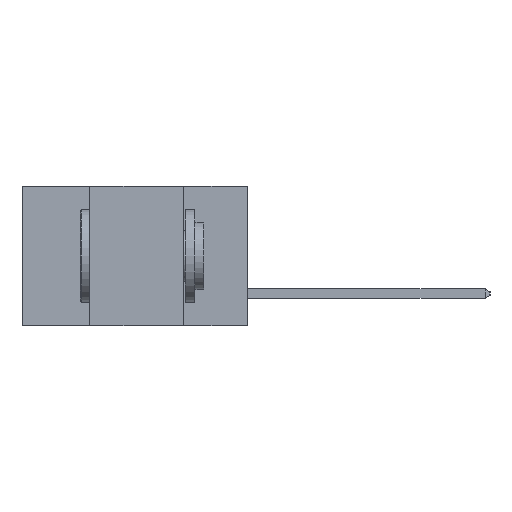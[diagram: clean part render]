
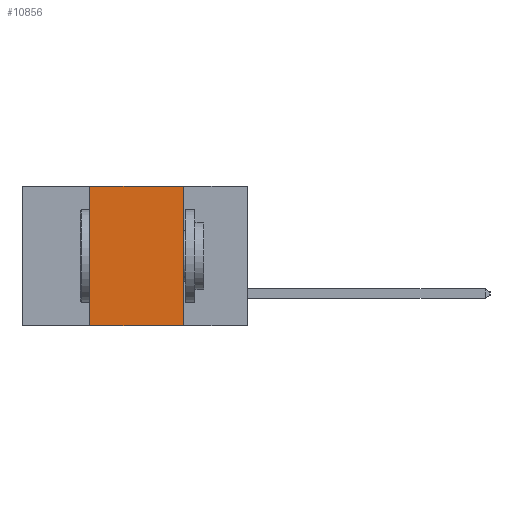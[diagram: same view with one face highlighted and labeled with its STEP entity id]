
A CAD part, left-side view. The second image highlights one B-rep face of the part: STEP entity #10856.
In plain terms, the highlighted planar face has unit normal (-1, 0, 0).
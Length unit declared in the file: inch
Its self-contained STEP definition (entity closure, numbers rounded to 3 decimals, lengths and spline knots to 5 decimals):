
#7 = CARTESIAN_POINT ( 'NONE',  ( 0., 0.6, 0. ) ) ;
#168 = ORIENTED_EDGE ( 'NONE', *, *, #8483, .F. ) ;
#930 = VECTOR ( 'NONE', #4495, 39.37008 ) ;
#2107 = CARTESIAN_POINT ( 'NONE',  ( 0., 0.17, 0. ) ) ;
#2740 = CARTESIAN_POINT ( 'NONE',  ( 0., 0.17, -0.37 ) ) ;
#2755 = DIRECTION ( 'NONE',  ( 0., 0., -1. ) ) ;
#2993 = EDGE_LOOP ( 'NONE', ( #13557, #168, #4222, #8613 ) ) ;
#3478 = EDGE_CURVE ( 'NONE', #11890, #4341, #4555, .T. ) ;
#3724 = VECTOR ( 'NONE', #5319, 39.37008 ) ;
#4222 = ORIENTED_EDGE ( 'NONE', *, *, #3478, .F. ) ;
#4341 = VERTEX_POINT ( 'NONE', #12393 ) ;
#4495 = DIRECTION ( 'NONE',  ( 0., 0., 1. ) ) ;
#4555 = LINE ( 'NONE', #6664, #930 ) ;
#5208 = CARTESIAN_POINT ( 'NONE',  ( 0., 0.42, -0.37 ) ) ;
#5319 = DIRECTION ( 'NONE',  ( 0., 0., -1. ) ) ;
#5603 = VERTEX_POINT ( 'NONE', #2740 ) ;
#6178 = EDGE_CURVE ( 'NONE', #11842, #5603, #11671, .T. ) ;
#6664 = CARTESIAN_POINT ( 'NONE',  ( 0., 0.42, 0. ) ) ;
#6954 = FACE_OUTER_BOUND ( 'NONE', #2993, .T. ) ;
#6997 = CARTESIAN_POINT ( 'NONE',  ( 0., 0.6, -0.37 ) ) ;
#7418 = VECTOR ( 'NONE', #13655, 39.37008 ) ;
#8483 = EDGE_CURVE ( 'NONE', #4341, #11842, #16281, .T. ) ;
#8613 = ORIENTED_EDGE ( 'NONE', *, *, #17142, .T. ) ;
#9283 = VECTOR ( 'NONE', #14559, 39.37008 ) ;
#9437 = PLANE ( 'NONE',  #10270 ) ;
#10270 = AXIS2_PLACEMENT_3D ( 'NONE', #7, #10788, #2755 ) ;
#10608 = CARTESIAN_POINT ( 'NONE',  ( 0., 0.6, 0. ) ) ;
#10788 = DIRECTION ( 'NONE',  ( 1., 0., 0. ) ) ;
#10856 = ADVANCED_FACE ( 'NONE', ( #6954 ), #9437, .F. ) ;
#10966 = LINE ( 'NONE', #6997, #7418 ) ;
#11671 = LINE ( 'NONE', #2107, #3724 ) ;
#11749 = CARTESIAN_POINT ( 'NONE',  ( 0., 0.17, 0. ) ) ;
#11842 = VERTEX_POINT ( 'NONE', #11749 ) ;
#11890 = VERTEX_POINT ( 'NONE', #5208 ) ;
#12393 = CARTESIAN_POINT ( 'NONE',  ( 0., 0.42, 0. ) ) ;
#13557 = ORIENTED_EDGE ( 'NONE', *, *, #6178, .F. ) ;
#13655 = DIRECTION ( 'NONE',  ( 0., -1., 0. ) ) ;
#14559 = DIRECTION ( 'NONE',  ( 0., -1., 0. ) ) ;
#16281 = LINE ( 'NONE', #10608, #9283 ) ;
#17142 = EDGE_CURVE ( 'NONE', #11890, #5603, #10966, .T. ) ;
